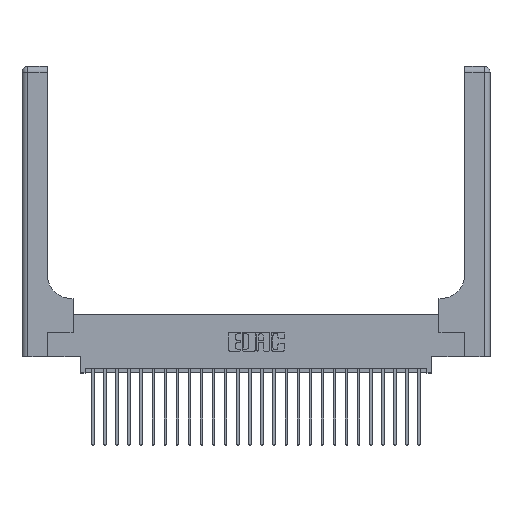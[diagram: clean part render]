
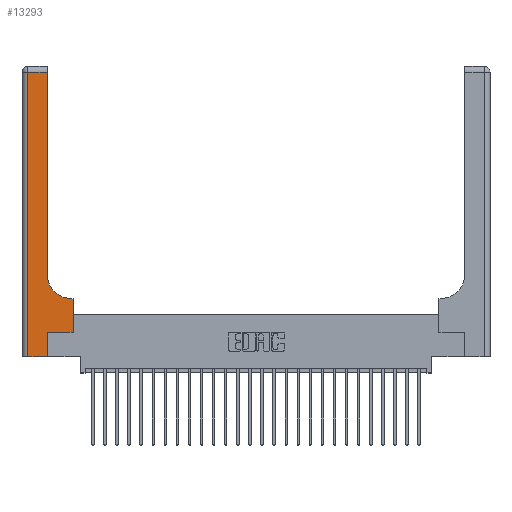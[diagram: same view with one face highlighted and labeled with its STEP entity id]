
A CAD part, top view. The second image highlights one B-rep face of the part: STEP entity #13293.
In plain terms, the highlighted planar face has unit normal (0, 0, 1).
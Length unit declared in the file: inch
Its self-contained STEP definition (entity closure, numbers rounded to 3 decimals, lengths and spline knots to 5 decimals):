
#125 = LINE ( 'NONE', #13135, #25076 ) ;
#327 = CIRCLE ( 'NONE', #2692, 0.25 ) ;
#601 = VERTEX_POINT ( 'NONE', #25071 ) ;
#708 = CARTESIAN_POINT ( 'NONE',  ( 0., 3., 0.37 ) ) ;
#1420 = CARTESIAN_POINT ( 'NONE',  ( 0.265, 0.25, 0.37 ) ) ;
#1494 = ORIENTED_EDGE ( 'NONE', *, *, #10226, .T. ) ;
#2220 = EDGE_CURVE ( 'NONE', #15058, #5718, #25072, .T. ) ;
#2356 = CARTESIAN_POINT ( 'NONE',  ( 0.51, 0.85, 0.37 ) ) ;
#2690 = AXIS2_PLACEMENT_3D ( 'NONE', #708, #2721, #16496 ) ;
#2692 = AXIS2_PLACEMENT_3D ( 'NONE', #2356, #16140, #4330 ) ;
#2721 = DIRECTION ( 'NONE',  ( 0., 0., -1. ) ) ;
#2949 = VERTEX_POINT ( 'NONE', #3774 ) ;
#3367 = CARTESIAN_POINT ( 'NONE',  ( 0.265, 0., 0.37 ) ) ;
#3774 = CARTESIAN_POINT ( 'NONE',  ( 0.26, 0.85, 0.37 ) ) ;
#4008 = ORIENTED_EDGE ( 'NONE', *, *, #13496, .T. ) ;
#4330 = DIRECTION ( 'NONE',  ( 1., 0., 0. ) ) ;
#4639 = VERTEX_POINT ( 'NONE', #1420 ) ;
#4694 = VECTOR ( 'NONE', #10479, 39.37008 ) ;
#4987 = CARTESIAN_POINT ( 'NONE',  ( 0.06, 2.94, 0.37 ) ) ;
#5228 = LINE ( 'NONE', #17635, #19696 ) ;
#5718 = VERTEX_POINT ( 'NONE', #20505 ) ;
#6087 = EDGE_CURVE ( 'NONE', #17554, #18002, #5228, .T. ) ;
#6290 = LINE ( 'NONE', #11952, #16141 ) ;
#7363 = VECTOR ( 'NONE', #10335, 39.37008 ) ;
#7432 = CARTESIAN_POINT ( 'NONE',  ( 0.528, 0.6, 0.37 ) ) ;
#7816 = DIRECTION ( 'NONE',  ( 1., 0., 0. ) ) ;
#8108 = CARTESIAN_POINT ( 'NONE',  ( 0.26, 3., 0.37 ) ) ;
#8710 = ORIENTED_EDGE ( 'NONE', *, *, #24579, .T. ) ;
#9324 = LINE ( 'NONE', #22274, #4694 ) ;
#9399 = VECTOR ( 'NONE', #13090, 39.37008 ) ;
#9857 = CARTESIAN_POINT ( 'NONE',  ( 0.06, 0., 0.37 ) ) ;
#10017 = VERTEX_POINT ( 'NONE', #25373 ) ;
#10226 = EDGE_CURVE ( 'NONE', #10017, #15058, #17843, .T. ) ;
#10293 = ORIENTED_EDGE ( 'NONE', *, *, #21754, .T. ) ;
#10335 = DIRECTION ( 'NONE',  ( 0., 1., 0. ) ) ;
#10408 = VERTEX_POINT ( 'NONE', #4987 ) ;
#10479 = DIRECTION ( 'NONE',  ( 1., 0., 0. ) ) ;
#11872 = EDGE_LOOP ( 'NONE', ( #10293, #16783, #4008, #22090, #24309, #8710, #1494, #25365, #15650 ) ) ;
#11952 = CARTESIAN_POINT ( 'NONE',  ( 0., 2.94, 0.37 ) ) ;
#13090 = DIRECTION ( 'NONE',  ( -1., 0., 0. ) ) ;
#13135 = CARTESIAN_POINT ( 'NONE',  ( 0.06, 3., 0.37 ) ) ;
#13190 = DIRECTION ( 'NONE',  ( 0., 1., 0. ) ) ;
#13204 = CARTESIAN_POINT ( 'NONE',  ( 0.26, 0.6, 0.37 ) ) ;
#13293 = ADVANCED_FACE ( 'NONE', ( #20813 ), #24292, .F. ) ;
#13496 = EDGE_CURVE ( 'NONE', #10408, #17554, #125, .T. ) ;
#14599 = LINE ( 'NONE', #3367, #19209 ) ;
#14641 = VECTOR ( 'NONE', #16039, 39.37008 ) ;
#15058 = VERTEX_POINT ( 'NONE', #7432 ) ;
#15526 = EDGE_CURVE ( 'NONE', #18002, #4639, #14599, .T. ) ;
#15650 = ORIENTED_EDGE ( 'NONE', *, *, #25187, .T. ) ;
#16039 = DIRECTION ( 'NONE',  ( 0., 1., 0. ) ) ;
#16140 = DIRECTION ( 'NONE',  ( 0., 0., -1. ) ) ;
#16141 = VECTOR ( 'NONE', #21824, 39.37008 ) ;
#16496 = DIRECTION ( 'NONE',  ( -1., 0., 0. ) ) ;
#16783 = ORIENTED_EDGE ( 'NONE', *, *, #23046, .T. ) ;
#17554 = VERTEX_POINT ( 'NONE', #9857 ) ;
#17635 = CARTESIAN_POINT ( 'NONE',  ( 0., 0., 0.37 ) ) ;
#17843 = LINE ( 'NONE', #22129, #7363 ) ;
#18002 = VERTEX_POINT ( 'NONE', #18891 ) ;
#18891 = CARTESIAN_POINT ( 'NONE',  ( 0.265, 0., 0.37 ) ) ;
#19209 = VECTOR ( 'NONE', #13190, 39.37008 ) ;
#19696 = VECTOR ( 'NONE', #7816, 39.37008 ) ;
#20505 = CARTESIAN_POINT ( 'NONE',  ( 0.51, 0.6, 0.37 ) ) ;
#20813 = FACE_OUTER_BOUND ( 'NONE', #11872, .T. ) ;
#20956 = DIRECTION ( 'NONE',  ( 0., -1., 0. ) ) ;
#21754 = EDGE_CURVE ( 'NONE', #2949, #601, #25062, .T. ) ;
#21824 = DIRECTION ( 'NONE',  ( -1., 0., 0. ) ) ;
#22090 = ORIENTED_EDGE ( 'NONE', *, *, #6087, .T. ) ;
#22129 = CARTESIAN_POINT ( 'NONE',  ( 0.528, 0.25, 0.37 ) ) ;
#22274 = CARTESIAN_POINT ( 'NONE',  ( 0.265, 0.25, 0.37 ) ) ;
#23046 = EDGE_CURVE ( 'NONE', #601, #10408, #6290, .T. ) ;
#24292 = PLANE ( 'NONE',  #2690 ) ;
#24309 = ORIENTED_EDGE ( 'NONE', *, *, #15526, .T. ) ;
#24579 = EDGE_CURVE ( 'NONE', #4639, #10017, #9324, .T. ) ;
#25062 = LINE ( 'NONE', #8108, #14641 ) ;
#25071 = CARTESIAN_POINT ( 'NONE',  ( 0.26, 2.94, 0.37 ) ) ;
#25072 = LINE ( 'NONE', #13204, #9399 ) ;
#25076 = VECTOR ( 'NONE', #20956, 39.37008 ) ;
#25187 = EDGE_CURVE ( 'NONE', #5718, #2949, #327, .T. ) ;
#25365 = ORIENTED_EDGE ( 'NONE', *, *, #2220, .T. ) ;
#25373 = CARTESIAN_POINT ( 'NONE',  ( 0.528, 0.25, 0.37 ) ) ;
